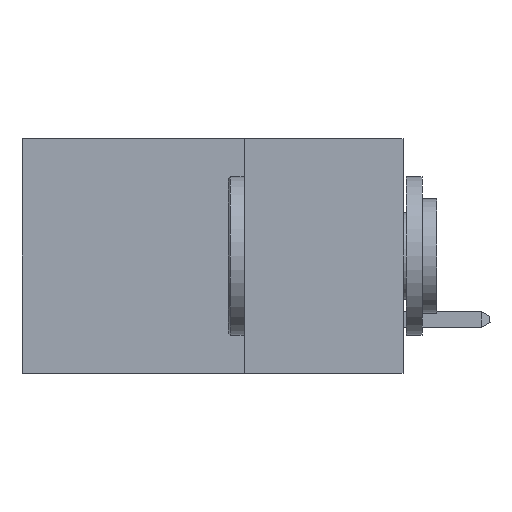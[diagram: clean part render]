
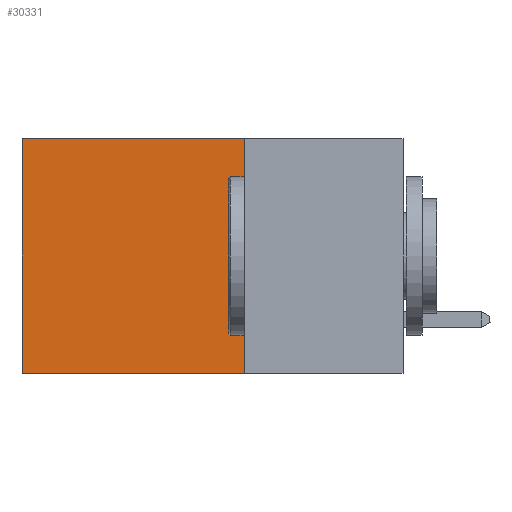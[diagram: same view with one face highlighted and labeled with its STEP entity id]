
A CAD part, left-side view. The second image highlights one B-rep face of the part: STEP entity #30331.
In plain terms, the highlighted planar face has unit normal (-1, 0, 0).
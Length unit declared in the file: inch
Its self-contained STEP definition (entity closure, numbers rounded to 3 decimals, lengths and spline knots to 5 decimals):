
#927 = EDGE_CURVE ( 'NONE', #30754, #32320, #31354, .T. ) ;
#1977 = CARTESIAN_POINT ( 'NONE',  ( 0.2875, 0.25, 0. ) ) ;
#2420 = ORIENTED_EDGE ( 'NONE', *, *, #15651, .T. ) ;
#2686 = CARTESIAN_POINT ( 'NONE',  ( 0.2875, 0.6, 0. ) ) ;
#3317 = DIRECTION ( 'NONE',  ( 0., 1., 0. ) ) ;
#4716 = ORIENTED_EDGE ( 'NONE', *, *, #23704, .F. ) ;
#6422 = CARTESIAN_POINT ( 'NONE',  ( 0.2875, 0.6, 0. ) ) ;
#6484 = VECTOR ( 'NONE', #22316, 39.37008 ) ;
#7801 = AXIS2_PLACEMENT_3D ( 'NONE', #1977, #36813, #17892 ) ;
#9940 = FACE_OUTER_BOUND ( 'NONE', #33870, .T. ) ;
#10864 = VECTOR ( 'NONE', #13836, 39.37008 ) ;
#13836 = DIRECTION ( 'NONE',  ( 0., 0., -1. ) ) ;
#14207 = CARTESIAN_POINT ( 'NONE',  ( 0.2875, 0.25, -0.37 ) ) ;
#14464 = ORIENTED_EDGE ( 'NONE', *, *, #927, .T. ) ;
#14556 = VERTEX_POINT ( 'NONE', #32262 ) ;
#14707 = PLANE ( 'NONE',  #7801 ) ;
#15266 = ORIENTED_EDGE ( 'NONE', *, *, #25653, .F. ) ;
#15651 = EDGE_CURVE ( 'NONE', #32320, #14556, #31747, .T. ) ;
#17892 = DIRECTION ( 'NONE',  ( 0., 0., -1. ) ) ;
#19938 = CARTESIAN_POINT ( 'NONE',  ( 0.2875, 0.25, 0. ) ) ;
#22316 = DIRECTION ( 'NONE',  ( 0., 0., -1. ) ) ;
#22554 = VERTEX_POINT ( 'NONE', #33710 ) ;
#22915 = VECTOR ( 'NONE', #3317, 39.37008 ) ;
#23704 = EDGE_CURVE ( 'NONE', #30754, #22554, #26705, .T. ) ;
#25653 = EDGE_CURVE ( 'NONE', #22554, #14556, #37199, .T. ) ;
#26705 = LINE ( 'NONE', #35945, #10864 ) ;
#26926 = DIRECTION ( 'NONE',  ( 0., 1., 0. ) ) ;
#28487 = CARTESIAN_POINT ( 'NONE',  ( 0.2875, 0.25, 0. ) ) ;
#28787 = VECTOR ( 'NONE', #26926, 39.37008 ) ;
#30331 = ADVANCED_FACE ( 'NONE', ( #9940 ), #14707, .F. ) ;
#30754 = VERTEX_POINT ( 'NONE', #19938 ) ;
#31354 = LINE ( 'NONE', #28487, #22915 ) ;
#31747 = LINE ( 'NONE', #6422, #6484 ) ;
#32262 = CARTESIAN_POINT ( 'NONE',  ( 0.2875, 0.6, -0.37 ) ) ;
#32320 = VERTEX_POINT ( 'NONE', #2686 ) ;
#33710 = CARTESIAN_POINT ( 'NONE',  ( 0.2875, 0.25, -0.37 ) ) ;
#33870 = EDGE_LOOP ( 'NONE', ( #2420, #15266, #4716, #14464 ) ) ;
#35945 = CARTESIAN_POINT ( 'NONE',  ( 0.2875, 0.25, 0. ) ) ;
#36813 = DIRECTION ( 'NONE',  ( 1., 0., 0. ) ) ;
#37199 = LINE ( 'NONE', #14207, #28787 ) ;
